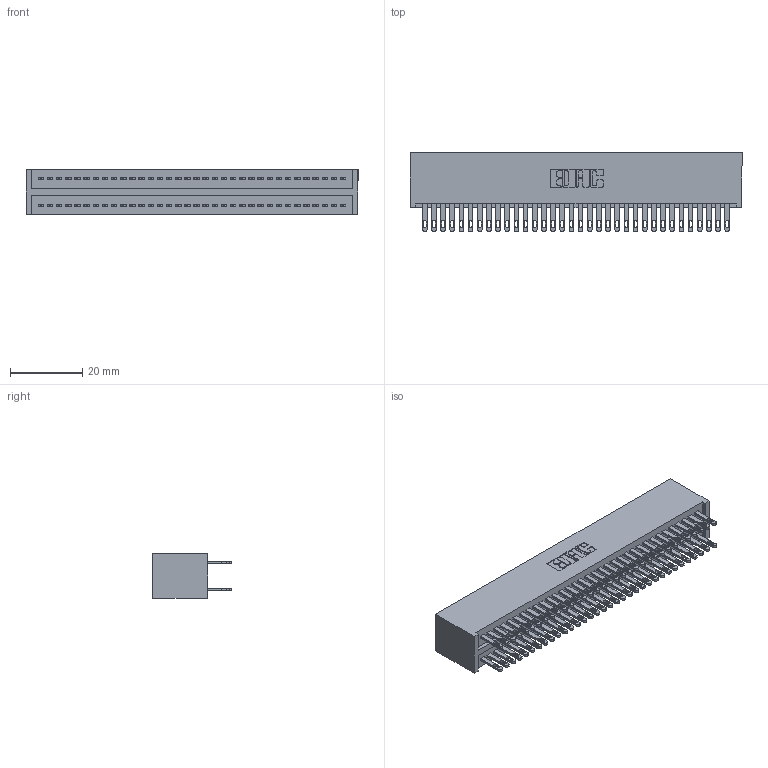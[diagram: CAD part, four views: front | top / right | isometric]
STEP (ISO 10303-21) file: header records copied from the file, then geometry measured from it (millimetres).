
FILE_DESCRIPTION (( 'STEP AP203' ), '1' );
FILE_NAME ('325-068-500-201.STEP', '2020-02-25T03:26:47', ( '' ), ( '' ), 'SwSTEP 2.0', 'SolidWorks 2016', '' );
FILE_SCHEMA (( 'CONFIG_CONTROL_DESIGN' ));
Length unit declared in the file: inch
Products named in the file (3): 325-068-500-201; 325 Part_Lugless; 325-292-001_325-293-100
Assembly tree (69 placements, depth 2):
  325-068-500-201
    325 Part_Lugless
    325-292-001_325-293-100  x68
Bounding box: 92 x 21.84 x 12.45 mm (x, y, z)
Volume: 12618.8 mm3; surface area: 16455.7 mm2
Topology: 69 solids, 69 shells, 3370 faces, 10283 edges, 6854 vertices
Faces by surface type: plane 2106, cylinder 1264
Entity records: 22561 total; most frequent: CARTESIAN_POINT 3746, ORIENTED_EDGE 3682, DIRECTION 3209, EDGE_CURVE 1841, VECTOR 1717, LINE 1717, VERTEX_POINT 1226, AXIS2_PLACEMENT_3D 746
